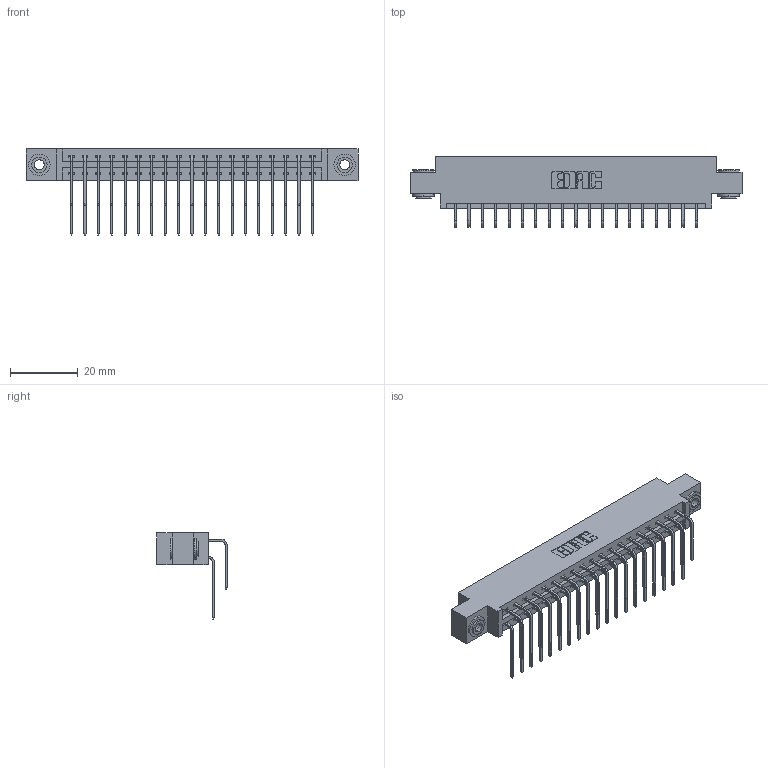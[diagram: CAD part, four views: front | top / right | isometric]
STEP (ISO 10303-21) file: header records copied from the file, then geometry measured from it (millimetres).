
FILE_DESCRIPTION (( 'STEP AP203' ), '1' );
FILE_NAME ('337-038-559-803.STEP', '2018-08-08T06:12:06', ( '' ), ( '' ), 'SwSTEP 2.0', 'SolidWorks 2016', '' );
FILE_SCHEMA (( 'CONFIG_CONTROL_DESIGN' ));
Length unit declared in the file: inch
Products named in the file (5): 345-250-002_345-250-002-102; 337-038-559-803; 337 Part_0.170 Offset - 0.156 Dia-TH; 345-292-001_558 559 Tail - 1; 345-292-001_559 Tail - 2
Assembly tree (41 placements, depth 2):
  337-038-559-803
    337 Part_0.170 Offset - 0.156 Dia-TH
    345-292-001_558 559 Tail - 1  x19
    345-292-001_559 Tail - 2  x19
    345-250-002_345-250-002-102  x2
Bounding box: 98.3 x 20.9 x 25.53 mm (x, y, z)
Volume: 10174.4 mm3; surface area: 12711.7 mm2
Topology: 41 solids, 41 shells, 2284 faces, 6745 edges, 4442 vertices
Faces by surface type: plane 1604, cylinder 672, cone 8
Entity records: 20272 total; most frequent: CARTESIAN_POINT 3456, ORIENTED_EDGE 3334, DIRECTION 2997, EDGE_CURVE 1667, VECTOR 1475, LINE 1475, VERTEX_POINT 1106, AXIS2_PLACEMENT_3D 761
